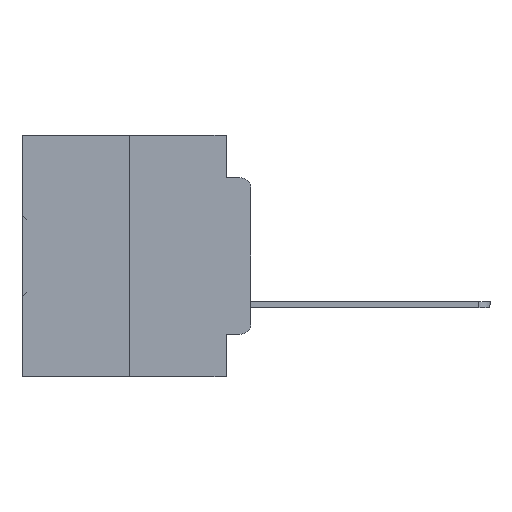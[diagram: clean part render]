
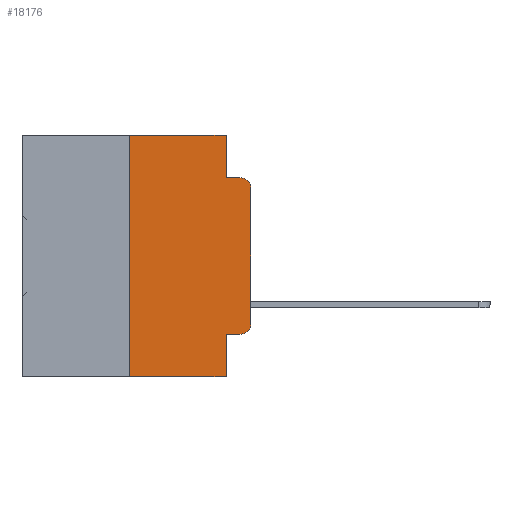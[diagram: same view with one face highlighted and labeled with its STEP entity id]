
A CAD part, left-side view. The second image highlights one B-rep face of the part: STEP entity #18176.
In plain terms, the highlighted planar face has unit normal (-1, 0, 0).
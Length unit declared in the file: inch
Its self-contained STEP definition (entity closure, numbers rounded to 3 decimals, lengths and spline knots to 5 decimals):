
#1346 = LINE ( 'NONE', #32923, #6252 ) ;
#1655 = LINE ( 'NONE', #4115, #8527 ) ;
#1788 = VERTEX_POINT ( 'NONE', #10886 ) ;
#1796 = PLANE ( 'NONE',  #30895 ) ;
#2246 = VECTOR ( 'NONE', #16970, 39.37008 ) ;
#2387 = DIRECTION ( 'NONE',  ( 0., 0., 1. ) ) ;
#3097 = EDGE_CURVE ( 'NONE', #16732, #1788, #17081, .T. ) ;
#3442 = CARTESIAN_POINT ( 'NONE',  ( 0., 0.051, -0.5 ) ) ;
#3823 = VERTEX_POINT ( 'NONE', #7122 ) ;
#4115 = CARTESIAN_POINT ( 'NONE',  ( 0., 0.051, -0.4115 ) ) ;
#4491 = CARTESIAN_POINT ( 'NONE',  ( 0., 0.051, -0.0885 ) ) ;
#4770 = DIRECTION ( 'NONE',  ( 0., 0., -1. ) ) ;
#4889 = VERTEX_POINT ( 'NONE', #18453 ) ;
#5230 = DIRECTION ( 'NONE',  ( 0., -1., 0. ) ) ;
#6126 = VERTEX_POINT ( 'NONE', #3442 ) ;
#6239 = LINE ( 'NONE', #19993, #2246 ) ;
#6252 = VECTOR ( 'NONE', #30094, 39.37008 ) ;
#6866 = CARTESIAN_POINT ( 'NONE',  ( 0., 0.051, 0. ) ) ;
#7122 = CARTESIAN_POINT ( 'NONE',  ( 0., 0.25, 0. ) ) ;
#7281 = EDGE_CURVE ( 'NONE', #11912, #36069, #6239, .T. ) ;
#7954 = ORIENTED_EDGE ( 'NONE', *, *, #19021, .T. ) ;
#8115 = CARTESIAN_POINT ( 'NONE',  ( 0., 0.473, -0.5 ) ) ;
#8495 = DIRECTION ( 'NONE',  ( -1., 0., 0. ) ) ;
#8527 = VECTOR ( 'NONE', #15189, 39.37008 ) ;
#8564 = ORIENTED_EDGE ( 'NONE', *, *, #17477, .T. ) ;
#8841 = LINE ( 'NONE', #23877, #26309 ) ;
#8967 = ORIENTED_EDGE ( 'NONE', *, *, #17875, .F. ) ;
#9505 = CARTESIAN_POINT ( 'NONE',  ( 0., 0.02, -0.4115 ) ) ;
#9712 = DIRECTION ( 'NONE',  ( -1., 0., 0. ) ) ;
#10426 = DIRECTION ( 'NONE',  ( 1., 0., 0. ) ) ;
#10562 = CIRCLE ( 'NONE', #18343, 0.02 ) ;
#10645 = EDGE_CURVE ( 'NONE', #23745, #6126, #29263, .T. ) ;
#10802 = ORIENTED_EDGE ( 'NONE', *, *, #20981, .T. ) ;
#10886 = CARTESIAN_POINT ( 'NONE',  ( 0., 0., -0.3915 ) ) ;
#11410 = ORIENTED_EDGE ( 'NONE', *, *, #3097, .T. ) ;
#11656 = VECTOR ( 'NONE', #2387, 39.37008 ) ;
#11771 = LINE ( 'NONE', #34325, #11656 ) ;
#11912 = VERTEX_POINT ( 'NONE', #20811 ) ;
#11968 = DIRECTION ( 'NONE',  ( 0., 0., -1. ) ) ;
#12854 = VECTOR ( 'NONE', #27859, 39.37008 ) ;
#13514 = ORIENTED_EDGE ( 'NONE', *, *, #28383, .T. ) ;
#14204 = CARTESIAN_POINT ( 'NONE',  ( 0., 0.051, -0.4115 ) ) ;
#15189 = DIRECTION ( 'NONE',  ( 0., -1., 0. ) ) ;
#16614 = ORIENTED_EDGE ( 'NONE', *, *, #22240, .F. ) ;
#16732 = VERTEX_POINT ( 'NONE', #9505 ) ;
#16970 = DIRECTION ( 'NONE',  ( 0., 0., -1. ) ) ;
#17081 = CIRCLE ( 'NONE', #20106, 0.02 ) ;
#17219 = CARTESIAN_POINT ( 'NONE',  ( 0., 0., -0.1085 ) ) ;
#17477 = EDGE_CURVE ( 'NONE', #18943, #6126, #37077, .T. ) ;
#17875 = EDGE_CURVE ( 'NONE', #18943, #3823, #11771, .T. ) ;
#18176 = ADVANCED_FACE ( 'NONE', ( #33362 ), #1796, .F. ) ;
#18343 = AXIS2_PLACEMENT_3D ( 'NONE', #26465, #9712, #21191 ) ;
#18453 = CARTESIAN_POINT ( 'NONE',  ( 0., 0.02, -0.0885 ) ) ;
#18943 = VERTEX_POINT ( 'NONE', #20101 ) ;
#18984 = ORIENTED_EDGE ( 'NONE', *, *, #24492, .F. ) ;
#19021 = EDGE_CURVE ( 'NONE', #33197, #4889, #10562, .T. ) ;
#19993 = CARTESIAN_POINT ( 'NONE',  ( 0., 0.051, 0. ) ) ;
#20101 = CARTESIAN_POINT ( 'NONE',  ( 0., 0.25, -0.5 ) ) ;
#20106 = AXIS2_PLACEMENT_3D ( 'NONE', #22075, #8495, #4770 ) ;
#20811 = CARTESIAN_POINT ( 'NONE',  ( 0., 0.051, 0. ) ) ;
#20981 = EDGE_CURVE ( 'NONE', #23745, #16732, #1655, .T. ) ;
#21191 = DIRECTION ( 'NONE',  ( 0., 0., -1. ) ) ;
#21914 = DIRECTION ( 'NONE',  ( 0., 0., -1. ) ) ;
#22075 = CARTESIAN_POINT ( 'NONE',  ( 0., 0.02, -0.3915 ) ) ;
#22240 = EDGE_CURVE ( 'NONE', #3823, #11912, #33787, .T. ) ;
#22461 = ORIENTED_EDGE ( 'NONE', *, *, #10645, .F. ) ;
#23689 = VECTOR ( 'NONE', #11968, 39.37008 ) ;
#23745 = VERTEX_POINT ( 'NONE', #14204 ) ;
#23877 = CARTESIAN_POINT ( 'NONE',  ( 0., 0., 0. ) ) ;
#24118 = VECTOR ( 'NONE', #5230, 39.37008 ) ;
#24492 = EDGE_CURVE ( 'NONE', #36069, #4889, #1346, .T. ) ;
#26309 = VECTOR ( 'NONE', #32159, 39.37008 ) ;
#26465 = CARTESIAN_POINT ( 'NONE',  ( 0., 0.02, -0.1085 ) ) ;
#27309 = EDGE_LOOP ( 'NONE', ( #13514, #7954, #18984, #32752, #16614, #8967, #8564, #22461, #10802, #11410 ) ) ;
#27859 = DIRECTION ( 'NONE',  ( 0., -1., 0. ) ) ;
#28383 = EDGE_CURVE ( 'NONE', #1788, #33197, #8841, .T. ) ;
#29263 = LINE ( 'NONE', #6866, #23689 ) ;
#30094 = DIRECTION ( 'NONE',  ( 0., -1., 0. ) ) ;
#30895 = AXIS2_PLACEMENT_3D ( 'NONE', #36168, #10426, #21914 ) ;
#32159 = DIRECTION ( 'NONE',  ( 0., 0., 1. ) ) ;
#32752 = ORIENTED_EDGE ( 'NONE', *, *, #7281, .F. ) ;
#32923 = CARTESIAN_POINT ( 'NONE',  ( 0., 0.051, -0.0885 ) ) ;
#33197 = VERTEX_POINT ( 'NONE', #17219 ) ;
#33362 = FACE_OUTER_BOUND ( 'NONE', #27309, .T. ) ;
#33428 = CARTESIAN_POINT ( 'NONE',  ( 0., 0.473, 0. ) ) ;
#33787 = LINE ( 'NONE', #33428, #24118 ) ;
#34325 = CARTESIAN_POINT ( 'NONE',  ( 0., 0.25, 0. ) ) ;
#36069 = VERTEX_POINT ( 'NONE', #4491 ) ;
#36168 = CARTESIAN_POINT ( 'NONE',  ( 0., 0.473, 0. ) ) ;
#37077 = LINE ( 'NONE', #8115, #12854 ) ;
